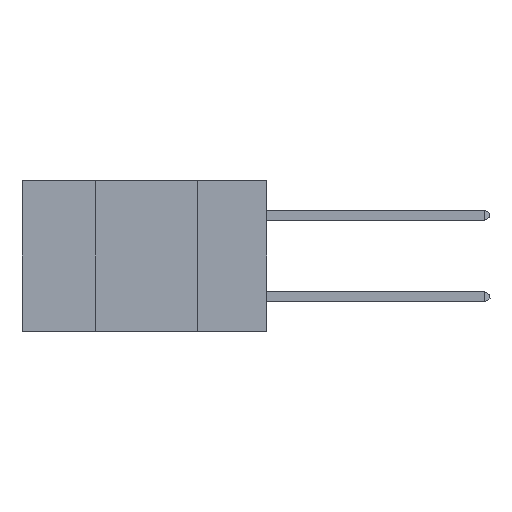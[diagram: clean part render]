
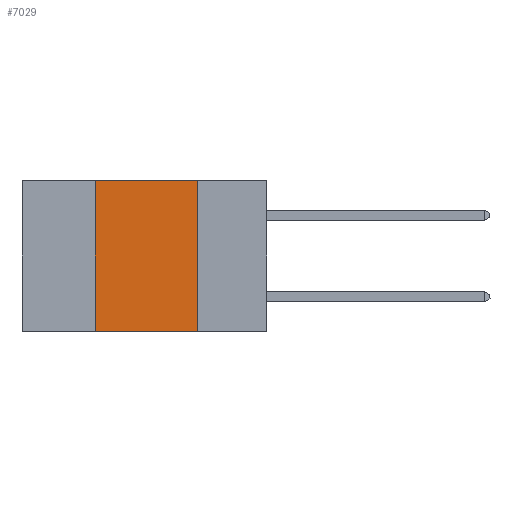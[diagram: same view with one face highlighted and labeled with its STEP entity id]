
A CAD part, left-side view. The second image highlights one B-rep face of the part: STEP entity #7029.
In plain terms, the highlighted planar face has unit normal (-1, 0, 0).
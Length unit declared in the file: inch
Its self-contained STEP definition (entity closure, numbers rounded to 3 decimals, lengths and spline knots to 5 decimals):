
#396 = CARTESIAN_POINT ( 'NONE',  ( 0., 0.17, -0.37 ) ) ;
#582 = CARTESIAN_POINT ( 'NONE',  ( 0., 0.6, 0. ) ) ;
#620 = DIRECTION ( 'NONE',  ( 1., 0., 0. ) ) ;
#630 = ORIENTED_EDGE ( 'NONE', *, *, #2063, .T. ) ;
#1584 = VERTEX_POINT ( 'NONE', #396 ) ;
#1997 = EDGE_CURVE ( 'NONE', #2080, #1584, #4432, .T. ) ;
#2063 = EDGE_CURVE ( 'NONE', #9383, #1584, #4291, .T. ) ;
#2080 = VERTEX_POINT ( 'NONE', #3584 ) ;
#2097 = CARTESIAN_POINT ( 'NONE',  ( 0., 0.42, 0. ) ) ;
#2201 = FACE_OUTER_BOUND ( 'NONE', #5406, .T. ) ;
#2264 = LINE ( 'NONE', #2097, #2624 ) ;
#2624 = VECTOR ( 'NONE', #6294, 39.37008 ) ;
#2955 = CARTESIAN_POINT ( 'NONE',  ( 0., 0.42, 0. ) ) ;
#3016 = DIRECTION ( 'NONE',  ( 0., -1., 0. ) ) ;
#3418 = CARTESIAN_POINT ( 'NONE',  ( 0., 0.17, 0. ) ) ;
#3584 = CARTESIAN_POINT ( 'NONE',  ( 0., 0.17, 0. ) ) ;
#3686 = VECTOR ( 'NONE', #3016, 39.37008 ) ;
#3801 = LINE ( 'NONE', #8368, #3686 ) ;
#4291 = LINE ( 'NONE', #9023, #6166 ) ;
#4432 = LINE ( 'NONE', #3418, #5174 ) ;
#4465 = CARTESIAN_POINT ( 'NONE',  ( 0., 0.42, -0.37 ) ) ;
#4589 = DIRECTION ( 'NONE',  ( 0., 0., -1. ) ) ;
#5019 = ORIENTED_EDGE ( 'NONE', *, *, #10019, .F. ) ;
#5021 = VERTEX_POINT ( 'NONE', #2955 ) ;
#5174 = VECTOR ( 'NONE', #8329, 39.37008 ) ;
#5406 = EDGE_LOOP ( 'NONE', ( #9488, #6119, #5019, #630 ) ) ;
#6103 = DIRECTION ( 'NONE',  ( 0., -1., 0. ) ) ;
#6119 = ORIENTED_EDGE ( 'NONE', *, *, #7681, .F. ) ;
#6166 = VECTOR ( 'NONE', #6103, 39.37008 ) ;
#6294 = DIRECTION ( 'NONE',  ( 0., 0., 1. ) ) ;
#7029 = ADVANCED_FACE ( 'NONE', ( #2201 ), #7108, .F. ) ;
#7108 = PLANE ( 'NONE',  #9329 ) ;
#7681 = EDGE_CURVE ( 'NONE', #5021, #2080, #3801, .T. ) ;
#8329 = DIRECTION ( 'NONE',  ( 0., 0., -1. ) ) ;
#8368 = CARTESIAN_POINT ( 'NONE',  ( 0., 0.6, 0. ) ) ;
#9023 = CARTESIAN_POINT ( 'NONE',  ( 0., 0.6, -0.37 ) ) ;
#9329 = AXIS2_PLACEMENT_3D ( 'NONE', #582, #620, #4589 ) ;
#9383 = VERTEX_POINT ( 'NONE', #4465 ) ;
#9488 = ORIENTED_EDGE ( 'NONE', *, *, #1997, .F. ) ;
#10019 = EDGE_CURVE ( 'NONE', #9383, #5021, #2264, .T. ) ;
